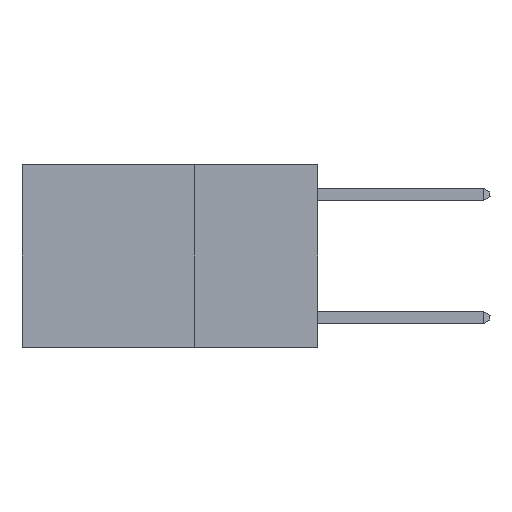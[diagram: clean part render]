
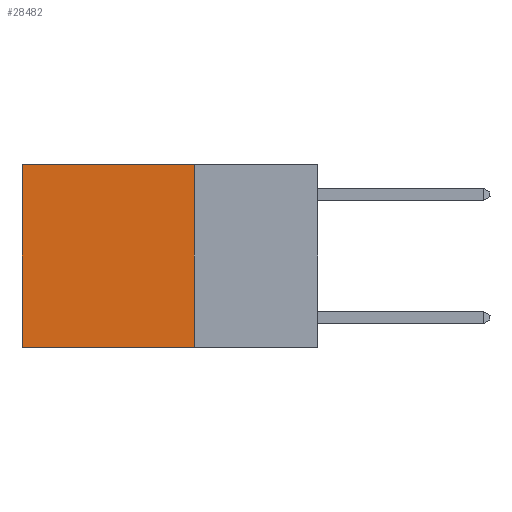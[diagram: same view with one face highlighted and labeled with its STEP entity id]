
A CAD part, left-side view. The second image highlights one B-rep face of the part: STEP entity #28482.
In plain terms, the highlighted planar face has unit normal (-1, 0, 0).
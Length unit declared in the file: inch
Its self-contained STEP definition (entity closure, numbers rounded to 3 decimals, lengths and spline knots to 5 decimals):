
#105 = CARTESIAN_POINT ( 'NONE',  ( 0.2625, 0.25, 0. ) ) ;
#613 = CARTESIAN_POINT ( 'NONE',  ( 0.2625, 0.6, -0.37 ) ) ;
#964 = DIRECTION ( 'NONE',  ( 1., 0., 0. ) ) ;
#1368 = EDGE_CURVE ( 'NONE', #4972, #1838, #28951, .T. ) ;
#1446 = VECTOR ( 'NONE', #25381, 39.37008 ) ;
#1838 = VERTEX_POINT ( 'NONE', #5029 ) ;
#2336 = ORIENTED_EDGE ( 'NONE', *, *, #29789, .F. ) ;
#4146 = EDGE_LOOP ( 'NONE', ( #12053, #19653, #2336, #6430 ) ) ;
#4936 = EDGE_CURVE ( 'NONE', #10653, #19510, #19350, .T. ) ;
#4972 = VERTEX_POINT ( 'NONE', #14637 ) ;
#5029 = CARTESIAN_POINT ( 'NONE',  ( 0.2625, 0.6, 0. ) ) ;
#5637 = DIRECTION ( 'NONE',  ( 0., 0., -1. ) ) ;
#6430 = ORIENTED_EDGE ( 'NONE', *, *, #1368, .T. ) ;
#6902 = VECTOR ( 'NONE', #5637, 39.37008 ) ;
#8161 = DIRECTION ( 'NONE',  ( 0., 0., -1. ) ) ;
#10653 = VERTEX_POINT ( 'NONE', #22297 ) ;
#10683 = CARTESIAN_POINT ( 'NONE',  ( 0.2625, 0.25, 0. ) ) ;
#10711 = PLANE ( 'NONE',  #16491 ) ;
#10725 = CARTESIAN_POINT ( 'NONE',  ( 0.2625, 0.6, 0. ) ) ;
#11201 = VECTOR ( 'NONE', #24243, 39.37008 ) ;
#12053 = ORIENTED_EDGE ( 'NONE', *, *, #25182, .T. ) ;
#14637 = CARTESIAN_POINT ( 'NONE',  ( 0.2625, 0.25, 0. ) ) ;
#14749 = DIRECTION ( 'NONE',  ( 0., 1., 0. ) ) ;
#16491 = AXIS2_PLACEMENT_3D ( 'NONE', #25309, #964, #8161 ) ;
#17076 = VECTOR ( 'NONE', #14749, 39.37008 ) ;
#17642 = LINE ( 'NONE', #105, #11201 ) ;
#19350 = LINE ( 'NONE', #22057, #17076 ) ;
#19510 = VERTEX_POINT ( 'NONE', #613 ) ;
#19653 = ORIENTED_EDGE ( 'NONE', *, *, #4936, .F. ) ;
#20861 = LINE ( 'NONE', #10725, #6902 ) ;
#22057 = CARTESIAN_POINT ( 'NONE',  ( 0.2625, 0.25, -0.37 ) ) ;
#22297 = CARTESIAN_POINT ( 'NONE',  ( 0.2625, 0.25, -0.37 ) ) ;
#24243 = DIRECTION ( 'NONE',  ( 0., 0., -1. ) ) ;
#25182 = EDGE_CURVE ( 'NONE', #1838, #19510, #20861, .T. ) ;
#25309 = CARTESIAN_POINT ( 'NONE',  ( 0.2625, 0.25, 0. ) ) ;
#25381 = DIRECTION ( 'NONE',  ( 0., 1., 0. ) ) ;
#28482 = ADVANCED_FACE ( 'NONE', ( #29795 ), #10711, .F. ) ;
#28951 = LINE ( 'NONE', #10683, #1446 ) ;
#29789 = EDGE_CURVE ( 'NONE', #4972, #10653, #17642, .T. ) ;
#29795 = FACE_OUTER_BOUND ( 'NONE', #4146, .T. ) ;
